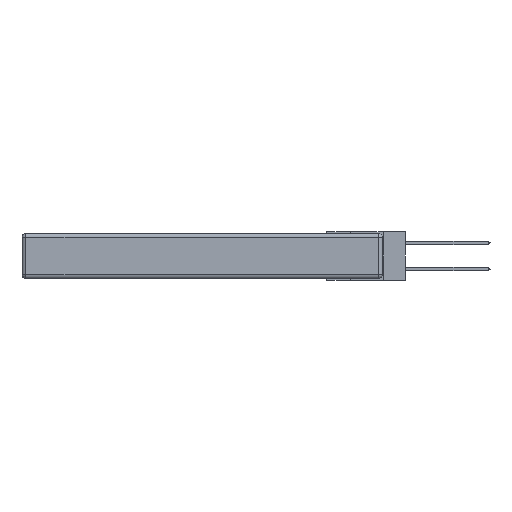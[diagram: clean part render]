
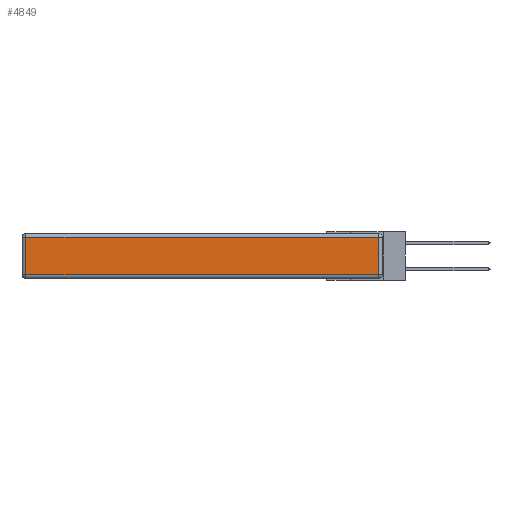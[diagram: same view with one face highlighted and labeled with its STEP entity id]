
A CAD part, left-side view. The second image highlights one B-rep face of the part: STEP entity #4849.
In plain terms, the highlighted planar face has unit normal (-1, 0, 0).
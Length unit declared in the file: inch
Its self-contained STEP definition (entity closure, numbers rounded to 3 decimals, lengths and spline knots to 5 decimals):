
#323 = CARTESIAN_POINT ( 'NONE',  ( 0., 2.72, -0.343 ) ) ;
#534 = VERTEX_POINT ( 'NONE', #8776 ) ;
#833 = AXIS2_PLACEMENT_3D ( 'NONE', #8428, #2994, #7459 ) ;
#1057 = EDGE_CURVE ( 'NONE', #534, #8087, #4007, .T. ) ;
#1377 = EDGE_CURVE ( 'NONE', #8948, #5497, #9561, .T. ) ;
#2165 = LINE ( 'NONE', #323, #3202 ) ;
#2417 = CARTESIAN_POINT ( 'NONE',  ( 0., 2.75, -0.03 ) ) ;
#2524 = DIRECTION ( 'NONE',  ( 0., 0., 1. ) ) ;
#2994 = DIRECTION ( 'NONE',  ( -1., 0., 0. ) ) ;
#3202 = VECTOR ( 'NONE', #5721, 39.37008 ) ;
#3494 = DIRECTION ( 'NONE',  ( 0., 1., 0. ) ) ;
#4007 = LINE ( 'NONE', #13971, #7123 ) ;
#4234 = VECTOR ( 'NONE', #2524, 39.37008 ) ;
#4849 = ADVANCED_FACE ( 'NONE', ( #11365 ), #7505, .T. ) ;
#5497 = VERTEX_POINT ( 'NONE', #9486 ) ;
#5635 = LINE ( 'NONE', #9020, #4234 ) ;
#5721 = DIRECTION ( 'NONE',  ( 0., 0., -1. ) ) ;
#7048 = EDGE_CURVE ( 'NONE', #8087, #8948, #5635, .T. ) ;
#7123 = VECTOR ( 'NONE', #7411, 39.37008 ) ;
#7411 = DIRECTION ( 'NONE',  ( 0., -1., 0. ) ) ;
#7459 = DIRECTION ( 'NONE',  ( 0., 0., 1. ) ) ;
#7505 = PLANE ( 'NONE',  #833 ) ;
#8087 = VERTEX_POINT ( 'NONE', #13783 ) ;
#8428 = CARTESIAN_POINT ( 'NONE',  ( 0., 0., -0.343 ) ) ;
#8567 = ORIENTED_EDGE ( 'NONE', *, *, #8823, .T. ) ;
#8776 = CARTESIAN_POINT ( 'NONE',  ( 0., 2.72, -0.313 ) ) ;
#8823 = EDGE_CURVE ( 'NONE', #5497, #534, #2165, .T. ) ;
#8948 = VERTEX_POINT ( 'NONE', #11358 ) ;
#9020 = CARTESIAN_POINT ( 'NONE',  ( 0., 0.03, -0.343 ) ) ;
#9486 = CARTESIAN_POINT ( 'NONE',  ( 0., 2.72, -0.03 ) ) ;
#9561 = LINE ( 'NONE', #2417, #11944 ) ;
#10092 = ORIENTED_EDGE ( 'NONE', *, *, #7048, .T. ) ;
#10399 = ORIENTED_EDGE ( 'NONE', *, *, #1057, .T. ) ;
#11358 = CARTESIAN_POINT ( 'NONE',  ( 0., 0.03, -0.03 ) ) ;
#11365 = FACE_OUTER_BOUND ( 'NONE', #12173, .T. ) ;
#11944 = VECTOR ( 'NONE', #3494, 39.37008 ) ;
#12173 = EDGE_LOOP ( 'NONE', ( #10399, #10092, #14119, #8567 ) ) ;
#13783 = CARTESIAN_POINT ( 'NONE',  ( 0., 0.03, -0.313 ) ) ;
#13971 = CARTESIAN_POINT ( 'NONE',  ( 0., 0., -0.313 ) ) ;
#14119 = ORIENTED_EDGE ( 'NONE', *, *, #1377, .T. ) ;
